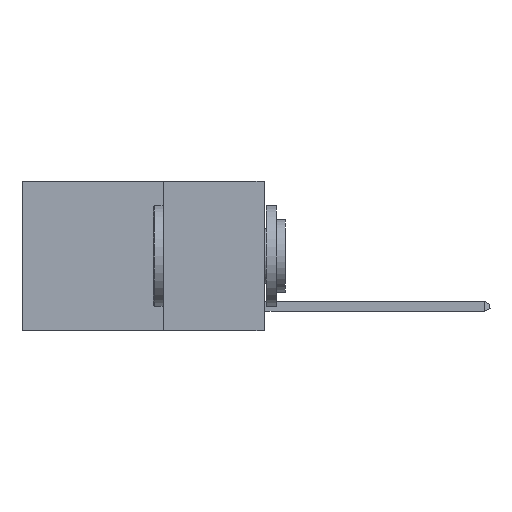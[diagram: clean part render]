
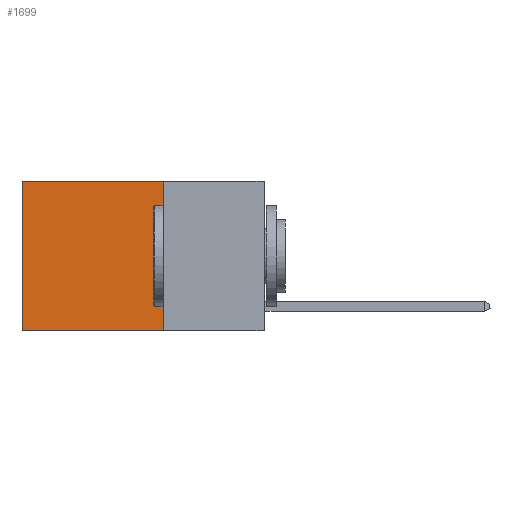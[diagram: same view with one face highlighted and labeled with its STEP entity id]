
A CAD part, left-side view. The second image highlights one B-rep face of the part: STEP entity #1699.
In plain terms, the highlighted planar face has unit normal (-1, 0, 0).
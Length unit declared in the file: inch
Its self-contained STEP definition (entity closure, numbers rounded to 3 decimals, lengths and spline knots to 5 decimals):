
#108 = VERTEX_POINT ( 'NONE', #8903 ) ;
#720 = CARTESIAN_POINT ( 'NONE',  ( 0.2625, 0.25, 0. ) ) ;
#814 = CARTESIAN_POINT ( 'NONE',  ( 0.2625, 0.6, -0.37 ) ) ;
#1204 = CARTESIAN_POINT ( 'NONE',  ( 0.2625, 0.6, 0. ) ) ;
#1309 = VECTOR ( 'NONE', #14615, 39.37008 ) ;
#1348 = EDGE_LOOP ( 'NONE', ( #7362, #5301, #2755, #3456 ) ) ;
#1699 = ADVANCED_FACE ( 'NONE', ( #13194 ), #2420, .F. ) ;
#2420 = PLANE ( 'NONE',  #2830 ) ;
#2755 = ORIENTED_EDGE ( 'NONE', *, *, #14275, .F. ) ;
#2830 = AXIS2_PLACEMENT_3D ( 'NONE', #12328, #12393, #3956 ) ;
#3456 = ORIENTED_EDGE ( 'NONE', *, *, #11910, .T. ) ;
#3956 = DIRECTION ( 'NONE',  ( 0., 0., -1. ) ) ;
#4461 = EDGE_CURVE ( 'NONE', #17808, #5808, #17155, .T. ) ;
#4801 = CARTESIAN_POINT ( 'NONE',  ( 0.2625, 0.25, -0.37 ) ) ;
#5301 = ORIENTED_EDGE ( 'NONE', *, *, #10603, .F. ) ;
#5808 = VERTEX_POINT ( 'NONE', #814 ) ;
#6157 = CARTESIAN_POINT ( 'NONE',  ( 0.2625, 0.25, -0.37 ) ) ;
#6523 = LINE ( 'NONE', #8991, #13608 ) ;
#7362 = ORIENTED_EDGE ( 'NONE', *, *, #4461, .T. ) ;
#7527 = DIRECTION ( 'NONE',  ( 0., 0., -1. ) ) ;
#8174 = LINE ( 'NONE', #720, #11530 ) ;
#8903 = CARTESIAN_POINT ( 'NONE',  ( 0.2625, 0.25, 0. ) ) ;
#8991 = CARTESIAN_POINT ( 'NONE',  ( 0.2625, 0.25, 0. ) ) ;
#10603 = EDGE_CURVE ( 'NONE', #18093, #5808, #12213, .T. ) ;
#11530 = VECTOR ( 'NONE', #12114, 39.37008 ) ;
#11910 = EDGE_CURVE ( 'NONE', #108, #17808, #6523, .T. ) ;
#12114 = DIRECTION ( 'NONE',  ( 0., 0., -1. ) ) ;
#12213 = LINE ( 'NONE', #6157, #1309 ) ;
#12328 = CARTESIAN_POINT ( 'NONE',  ( 0.2625, 0.25, 0. ) ) ;
#12393 = DIRECTION ( 'NONE',  ( 1., 0., 0. ) ) ;
#12907 = VECTOR ( 'NONE', #7527, 39.37008 ) ;
#13194 = FACE_OUTER_BOUND ( 'NONE', #1348, .T. ) ;
#13608 = VECTOR ( 'NONE', #14633, 39.37008 ) ;
#14275 = EDGE_CURVE ( 'NONE', #108, #18093, #8174, .T. ) ;
#14571 = CARTESIAN_POINT ( 'NONE',  ( 0.2625, 0.6, 0. ) ) ;
#14615 = DIRECTION ( 'NONE',  ( 0., 1., 0. ) ) ;
#14633 = DIRECTION ( 'NONE',  ( 0., 1., 0. ) ) ;
#17155 = LINE ( 'NONE', #14571, #12907 ) ;
#17808 = VERTEX_POINT ( 'NONE', #1204 ) ;
#18093 = VERTEX_POINT ( 'NONE', #4801 ) ;
